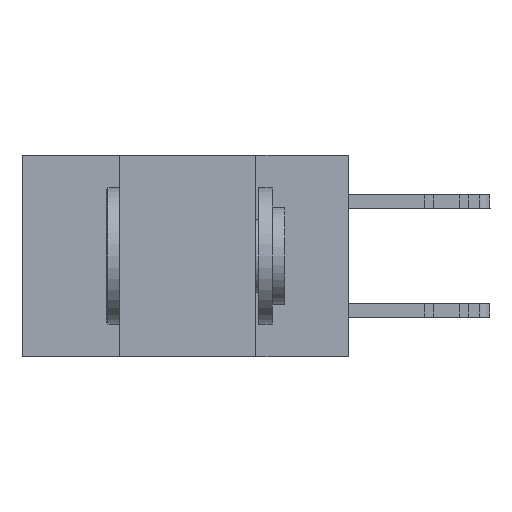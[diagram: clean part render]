
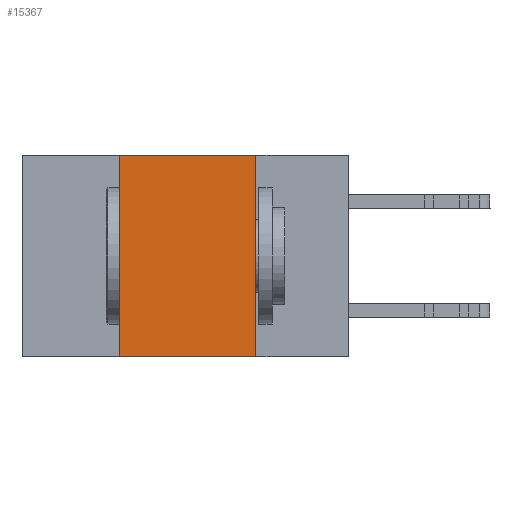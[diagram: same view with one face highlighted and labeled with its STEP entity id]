
A CAD part, left-side view. The second image highlights one B-rep face of the part: STEP entity #15367.
In plain terms, the highlighted planar face has unit normal (-1, 0, 0).
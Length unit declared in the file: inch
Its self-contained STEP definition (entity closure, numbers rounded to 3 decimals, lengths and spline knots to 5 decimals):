
#1740 = ORIENTED_EDGE ( 'NONE', *, *, #18889, .F. ) ;
#1994 = LINE ( 'NONE', #9708, #3544 ) ;
#2221 = DIRECTION ( 'NONE',  ( 1., 0., 0. ) ) ;
#2380 = VECTOR ( 'NONE', #11492, 39.37008 ) ;
#2850 = VECTOR ( 'NONE', #12257, 39.37008 ) ;
#2882 = EDGE_CURVE ( 'NONE', #13688, #20979, #1994, .T. ) ;
#3544 = VECTOR ( 'NONE', #9584, 39.37008 ) ;
#3638 = CARTESIAN_POINT ( 'NONE',  ( 0., 0.6, -0.37 ) ) ;
#3805 = CARTESIAN_POINT ( 'NONE',  ( 0., 0.17, -0.37 ) ) ;
#4651 = CARTESIAN_POINT ( 'NONE',  ( 0., 0.42, -0.37 ) ) ;
#4996 = CARTESIAN_POINT ( 'NONE',  ( 0., 0.17, 0. ) ) ;
#5119 = VERTEX_POINT ( 'NONE', #23613 ) ;
#6052 = FACE_OUTER_BOUND ( 'NONE', #16899, .T. ) ;
#7693 = PLANE ( 'NONE',  #15235 ) ;
#8299 = ORIENTED_EDGE ( 'NONE', *, *, #14612, .F. ) ;
#9043 = DIRECTION ( 'NONE',  ( 0., 0., -1. ) ) ;
#9292 = LINE ( 'NONE', #3805, #24112 ) ;
#9417 = VERTEX_POINT ( 'NONE', #23722 ) ;
#9584 = DIRECTION ( 'NONE',  ( 0., -1., 0. ) ) ;
#9708 = CARTESIAN_POINT ( 'NONE',  ( 0., 0.6, 0. ) ) ;
#9812 = DIRECTION ( 'NONE',  ( 0., 0., -1. ) ) ;
#11492 = DIRECTION ( 'NONE',  ( 0., -1., 0. ) ) ;
#11686 = CARTESIAN_POINT ( 'NONE',  ( 0., 0.6, 0. ) ) ;
#12059 = EDGE_CURVE ( 'NONE', #9417, #5119, #24025, .T. ) ;
#12072 = CARTESIAN_POINT ( 'NONE',  ( 0., 0.42, 0. ) ) ;
#12257 = DIRECTION ( 'NONE',  ( 0., 0., 1. ) ) ;
#13688 = VERTEX_POINT ( 'NONE', #12072 ) ;
#14612 = EDGE_CURVE ( 'NONE', #9417, #13688, #21915, .T. ) ;
#15235 = AXIS2_PLACEMENT_3D ( 'NONE', #11686, #2221, #9812 ) ;
#15367 = ADVANCED_FACE ( 'NONE', ( #6052 ), #7693, .F. ) ;
#16899 = EDGE_LOOP ( 'NONE', ( #1740, #19058, #8299, #24249 ) ) ;
#18889 = EDGE_CURVE ( 'NONE', #20979, #5119, #9292, .T. ) ;
#19058 = ORIENTED_EDGE ( 'NONE', *, *, #2882, .F. ) ;
#20979 = VERTEX_POINT ( 'NONE', #4996 ) ;
#21915 = LINE ( 'NONE', #4651, #2850 ) ;
#23613 = CARTESIAN_POINT ( 'NONE',  ( 0., 0.17, -0.37 ) ) ;
#23722 = CARTESIAN_POINT ( 'NONE',  ( 0., 0.42, -0.37 ) ) ;
#24025 = LINE ( 'NONE', #3638, #2380 ) ;
#24112 = VECTOR ( 'NONE', #9043, 39.37008 ) ;
#24249 = ORIENTED_EDGE ( 'NONE', *, *, #12059, .T. ) ;
